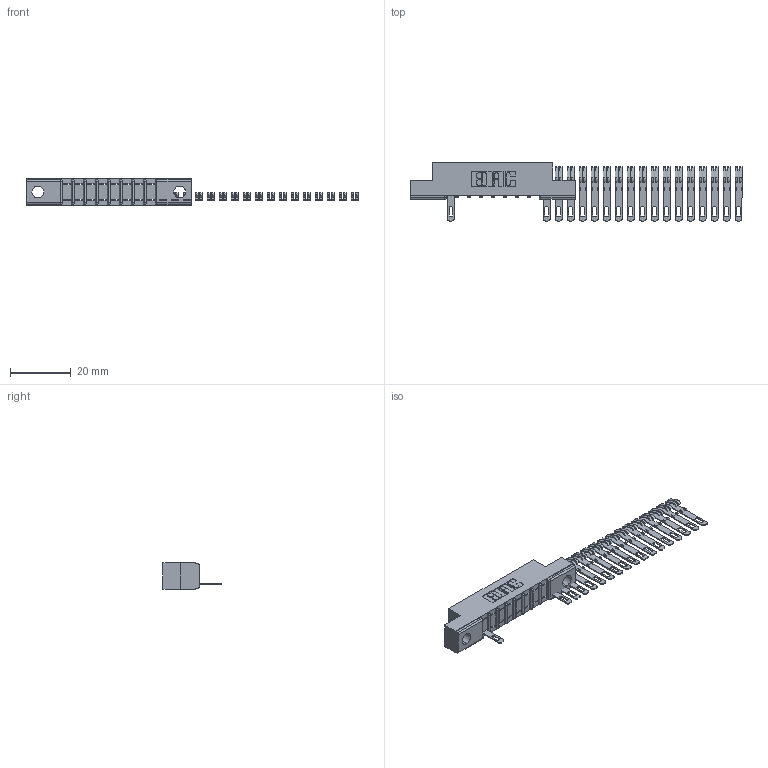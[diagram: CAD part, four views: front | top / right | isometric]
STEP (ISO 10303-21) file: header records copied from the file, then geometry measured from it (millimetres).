
FILE_DESCRIPTION (( 'STEP AP203' ), '1' );
FILE_NAME ('357-025-505-102.STEP', '2018-08-09T01:28:50', ( '' ), ( '' ), 'SwSTEP 2.0', 'SolidWorks 2016', '' );
FILE_SCHEMA (( 'CONFIG_CONTROL_DESIGN' ));
Length unit declared in the file: inch
Products named in the file (3): 307 Part_.128 Dia Mounting Holes; 307-290-001_505; 357-025-505-102
Assembly tree (19 placements, depth 2):
  357-025-505-102
    307 Part_.128 Dia Mounting Holes
    307-290-001_505  x18
Bounding box: 109.72 x 19.18 x 8.71 mm (x, y, z)
Volume: 3570.7 mm3; surface area: 5867.9 mm2
Topology: 19 solids, 19 shells, 935 faces, 2599 edges, 1682 vertices
Faces by surface type: plane 598, cylinder 319, sphere 18
Entity records: 11346 total; most frequent: CARTESIAN_POINT 1854, DIRECTION 1835, ORIENTED_EDGE 1830, EDGE_CURVE 915, LINE 685, VECTOR 685, VERTEX_POINT 594, AXIS2_PLACEMENT_3D 575
